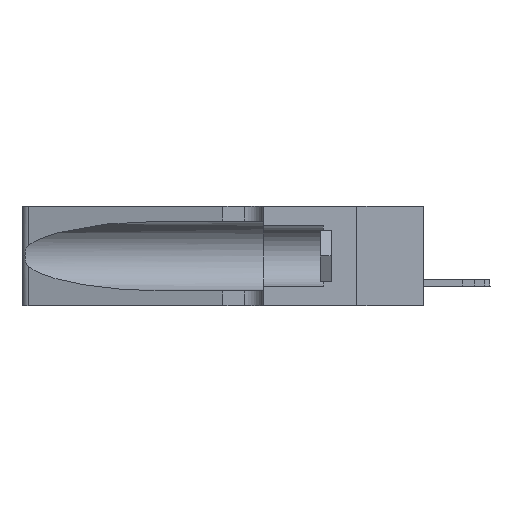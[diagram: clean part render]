
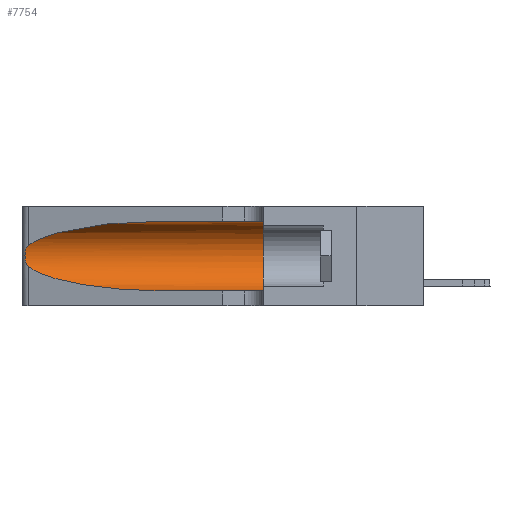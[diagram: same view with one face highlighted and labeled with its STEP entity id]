
A CAD part, left-side view. The second image highlights one B-rep face of the part: STEP entity #7754.
In plain terms, the highlighted cylindrical face has radius 3.308 mm (diameter 6.617 mm), a partial arc.
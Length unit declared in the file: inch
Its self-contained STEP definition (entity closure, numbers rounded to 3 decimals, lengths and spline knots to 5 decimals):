
#254 = CARTESIAN_POINT ( 'NONE',  ( 0.25856, 1.23593, 0.16098 ) ) ;
#2454 = CARTESIAN_POINT ( 'NONE',  ( 0.2373, 1.15595, 0.08982 ) ) ;
#2881 = CARTESIAN_POINT ( 'NONE',  ( 0.1305, 1.61858, 0.31525 ) ) ;
#3046 = ORIENTED_EDGE ( 'NONE', *, *, #34642, .T. ) ;
#3259 = CARTESIAN_POINT ( 'NONE',  ( 0.1305, 0.72297, 0.05475 ) ) ;
#3465 = VERTEX_POINT ( 'NONE', #18443 ) ;
#3958 = CARTESIAN_POINT ( 'NONE',  ( 0.26018, 1.23835, 0.19895 ) ) ;
#5476 =( BOUNDED_CURVE ( )  B_SPLINE_CURVE ( 3, ( #32899, #12315, #14649, #8344 ),
 .UNSPECIFIED., .F., .F. ) 
 B_SPLINE_CURVE_WITH_KNOTS ( ( 4, 4 ),
 ( 1.5708, 2.84003 ),
 .UNSPECIFIED. ) 
 CURVE ( )  GEOMETRIC_REPRESENTATION_ITEM ( )  RATIONAL_B_SPLINE_CURVE ( ( 1., 0.87, 0.87, 1. ) ) 
 REPRESENTATION_ITEM ( '' )  );
#5621 = CYLINDRICAL_SURFACE ( 'NONE', #35331, 0.13025 ) ;
#5892 = DIRECTION ( 'NONE',  ( 0., 1., 0. ) ) ;
#7593 = CARTESIAN_POINT ( 'NONE',  ( 0.25487, 1.22718, 0.22369 ) ) ;
#7754 = ADVANCED_FACE ( 'NONE', ( #33023 ), #5621, .F. ) ;
#8344 = CARTESIAN_POINT ( 'NONE',  ( 0.25487, 1.22718, 0.22369 ) ) ;
#8651 = VECTOR ( 'NONE', #27691, 39.37008 ) ;
#9192 = CARTESIAN_POINT ( 'NONE',  ( 0.25789, 1.23486, 0.15765 ) ) ;
#10076 = CARTESIAN_POINT ( 'NONE',  ( 0.25487, 1.22718, 0.22369 ) ) ;
#11311 = EDGE_CURVE ( 'NONE', #32435, #24320, #5476, .T. ) ;
#12147 = CARTESIAN_POINT ( 'NONE',  ( 0.25555, 1.22994, 0.2215 ) ) ;
#12315 = CARTESIAN_POINT ( 'NONE',  ( 0.18966, 0.96281, 0.31525 ) ) ;
#14046 = EDGE_CURVE ( 'NONE', #3465, #27597, #20812, .T. ) ;
#14646 = CARTESIAN_POINT ( 'NONE',  ( 0.1305, 0.72297, 0.05475 ) ) ;
#14649 = CARTESIAN_POINT ( 'NONE',  ( 0.2373, 1.15595, 0.28018 ) ) ;
#14715 = ORIENTED_EDGE ( 'NONE', *, *, #14046, .F. ) ;
#15114 = CARTESIAN_POINT ( 'NONE',  ( 0.25854, 1.2359, 0.20912 ) ) ;
#15213 = EDGE_LOOP ( 'NONE', ( #19491, #3046, #20219, #21963, #14715, #16851 ) ) ;
#15746 = CARTESIAN_POINT ( 'NONE',  ( 0.25487, 1.22718, 0.14631 ) ) ;
#15763 = EDGE_CURVE ( 'NONE', #32435, #3465, #25352, .T. ) ;
#16851 = ORIENTED_EDGE ( 'NONE', *, *, #15763, .F. ) ;
#17627 = DIRECTION ( 'NONE',  ( 0., 0., -1. ) ) ;
#18443 = CARTESIAN_POINT ( 'NONE',  ( 0.1305, 0.35, 0.31525 ) ) ;
#19147 = AXIS2_PLACEMENT_3D ( 'NONE', #36419, #5892, #24270 ) ;
#19491 = ORIENTED_EDGE ( 'NONE', *, *, #11311, .T. ) ;
#20051 = VERTEX_POINT ( 'NONE', #3259 ) ;
#20219 = ORIENTED_EDGE ( 'NONE', *, *, #33310, .T. ) ;
#20812 = CIRCLE ( 'NONE', #19147, 0.13025 ) ;
#21083 = CARTESIAN_POINT ( 'NONE',  ( 0.26075, 1.23896, 0.178 ) ) ;
#21183 = EDGE_CURVE ( 'NONE', #20051, #27597, #32952, .T. ) ;
#21400 = CARTESIAN_POINT ( 'NONE',  ( 0.1305, 1.61858, 0.05475 ) ) ;
#21963 = ORIENTED_EDGE ( 'NONE', *, *, #21183, .T. ) ;
#23278 =( BOUNDED_CURVE ( )  B_SPLINE_CURVE ( 3, ( #23716, #2454, #26639, #14646 ),
 .UNSPECIFIED., .F., .T. ) 
 B_SPLINE_CURVE_WITH_KNOTS ( ( 4, 4 ),
 ( 3.44316, 4.71239 ),
 .UNSPECIFIED. ) 
 CURVE ( )  GEOMETRIC_REPRESENTATION_ITEM ( )  RATIONAL_B_SPLINE_CURVE ( ( 1., 0.87, 0.87, 1. ) ) 
 REPRESENTATION_ITEM ( '' )  );
#23716 = CARTESIAN_POINT ( 'NONE',  ( 0.25487, 1.22718, 0.14631 ) ) ;
#24270 = DIRECTION ( 'NONE',  ( 0., 0., 1. ) ) ;
#24320 = VERTEX_POINT ( 'NONE', #7593 ) ;
#24591 = CARTESIAN_POINT ( 'NONE',  ( 0.25639, 1.23186, 0.15144 ) ) ;
#24996 = VECTOR ( 'NONE', #30171, 39.37008 ) ;
#25352 = LINE ( 'NONE', #2881, #8651 ) ;
#26639 = CARTESIAN_POINT ( 'NONE',  ( 0.18966, 0.96281, 0.05475 ) ) ;
#27597 = VERTEX_POINT ( 'NONE', #35039 ) ;
#27691 = DIRECTION ( 'NONE',  ( 0., -1., 0. ) ) ;
#27856 = CARTESIAN_POINT ( 'NONE',  ( 0.25487, 1.22718, 0.14631 ) ) ;
#27912 = CARTESIAN_POINT ( 'NONE',  ( 0.25555, 1.22993, 0.14849 ) ) ;
#30171 = DIRECTION ( 'NONE',  ( 0., -1., 0. ) ) ;
#30880 = CARTESIAN_POINT ( 'NONE',  ( 0.26017, 1.23833, 0.17102 ) ) ;
#31027 = CARTESIAN_POINT ( 'NONE',  ( 0.25787, 1.23484, 0.2124 ) ) ;
#32435 = VERTEX_POINT ( 'NONE', #37376 ) ;
#32899 = CARTESIAN_POINT ( 'NONE',  ( 0.1305, 0.72297, 0.31525 ) ) ;
#32952 = LINE ( 'NONE', #21400, #24996 ) ;
#33023 = FACE_OUTER_BOUND ( 'NONE', #15213, .T. ) ;
#33310 = EDGE_CURVE ( 'NONE', #36734, #20051, #23278, .T. ) ;
#34642 = EDGE_CURVE ( 'NONE', #24320, #36734, #38379, .T. ) ;
#35039 = CARTESIAN_POINT ( 'NONE',  ( 0.1305, 0.35, 0.05475 ) ) ;
#35331 = AXIS2_PLACEMENT_3D ( 'NONE', #35503, #38127, #17627 ) ;
#35503 = CARTESIAN_POINT ( 'NONE',  ( 0.1305, 1.61858, 0.185 ) ) ;
#35991 = CARTESIAN_POINT ( 'NONE',  ( 0.26075, 1.23896, 0.19203 ) ) ;
#36419 = CARTESIAN_POINT ( 'NONE',  ( 0.1305, 0.35, 0.185 ) ) ;
#36617 = CARTESIAN_POINT ( 'NONE',  ( 0.25639, 1.23184, 0.21858 ) ) ;
#36734 = VERTEX_POINT ( 'NONE', #27856 ) ;
#37376 = CARTESIAN_POINT ( 'NONE',  ( 0.1305, 0.72297, 0.31525 ) ) ;
#38127 = DIRECTION ( 'NONE',  ( 0., -1., 0. ) ) ;
#38379 = B_SPLINE_CURVE_WITH_KNOTS ( 'NONE', 3,
 ( #10076, #12147, #36617, #31027, #15114, #3958, #35991, #21083, #30880, #254, #9192, #24591, #27912, #15746 ),
 .UNSPECIFIED., .F., .F.,
 ( 4, 2, 2, 2, 2, 2, 4 ),
 ( 0., 0.00027, 0.00053, 0.00107, 0.0016, 0.00187, 0.00214 ),
 .UNSPECIFIED. ) ;
